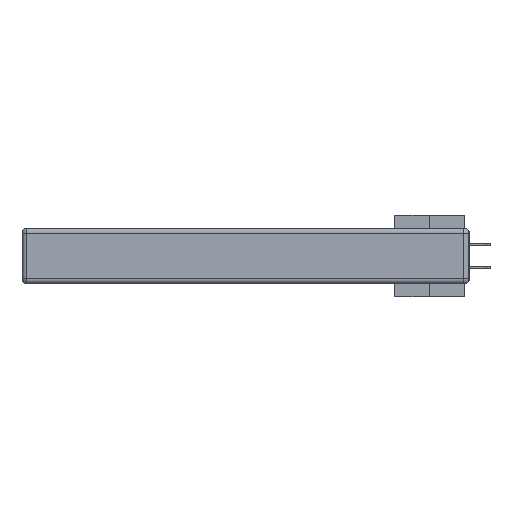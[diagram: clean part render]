
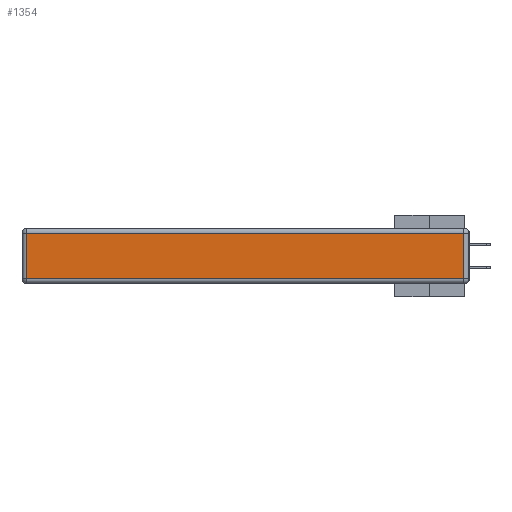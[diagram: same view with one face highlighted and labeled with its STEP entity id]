
A CAD part, left-side view. The second image highlights one B-rep face of the part: STEP entity #1354.
In plain terms, the highlighted planar face has unit normal (-1, 0, 0).
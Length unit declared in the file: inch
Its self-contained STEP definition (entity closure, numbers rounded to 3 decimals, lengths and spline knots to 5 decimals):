
#1354 = ADVANCED_FACE ( 'NONE', ( #19549 ), #22394, .T. ) ;
#1732 = EDGE_CURVE ( 'NONE', #22104, #39568, #37034, .T. ) ;
#2135 = VECTOR ( 'NONE', #3026, 39.37008 ) ;
#3026 = DIRECTION ( 'NONE',  ( 0., 1., 0. ) ) ;
#4450 = CARTESIAN_POINT ( 'NONE',  ( 0., 0.03, -0.313 ) ) ;
#4521 = CARTESIAN_POINT ( 'NONE',  ( 0., 2.72, -0.343 ) ) ;
#7604 = VERTEX_POINT ( 'NONE', #21074 ) ;
#8229 = AXIS2_PLACEMENT_3D ( 'NONE', #32051, #25881, #12905 ) ;
#12905 = DIRECTION ( 'NONE',  ( 0., 0., 1. ) ) ;
#13509 = VECTOR ( 'NONE', #14824, 39.37008 ) ;
#14205 = EDGE_CURVE ( 'NONE', #39568, #21050, #15308, .T. ) ;
#14693 = ORIENTED_EDGE ( 'NONE', *, *, #22444, .T. ) ;
#14824 = DIRECTION ( 'NONE',  ( 0., -1., 0. ) ) ;
#15308 = LINE ( 'NONE', #20934, #35846 ) ;
#17295 = DIRECTION ( 'NONE',  ( 0., 0., 1. ) ) ;
#17671 = CARTESIAN_POINT ( 'NONE',  ( 0., 0., -0.313 ) ) ;
#19263 = CARTESIAN_POINT ( 'NONE',  ( 0., 0.03, -0.03 ) ) ;
#19549 = FACE_OUTER_BOUND ( 'NONE', #19944, .T. ) ;
#19944 = EDGE_LOOP ( 'NONE', ( #39449, #34553, #14693, #27060 ) ) ;
#20934 = CARTESIAN_POINT ( 'NONE',  ( 0., 0.03, -0.343 ) ) ;
#21050 = VERTEX_POINT ( 'NONE', #19263 ) ;
#21074 = CARTESIAN_POINT ( 'NONE',  ( 0., 2.72, -0.03 ) ) ;
#22104 = VERTEX_POINT ( 'NONE', #36295 ) ;
#22394 = PLANE ( 'NONE',  #8229 ) ;
#22444 = EDGE_CURVE ( 'NONE', #21050, #7604, #39155, .T. ) ;
#23056 = VECTOR ( 'NONE', #29343, 39.37008 ) ;
#24532 = LINE ( 'NONE', #4521, #23056 ) ;
#25881 = DIRECTION ( 'NONE',  ( -1., 0., 0. ) ) ;
#27060 = ORIENTED_EDGE ( 'NONE', *, *, #31257, .T. ) ;
#28526 = CARTESIAN_POINT ( 'NONE',  ( 0., 2.75, -0.03 ) ) ;
#29343 = DIRECTION ( 'NONE',  ( 0., 0., -1. ) ) ;
#31257 = EDGE_CURVE ( 'NONE', #7604, #22104, #24532, .T. ) ;
#32051 = CARTESIAN_POINT ( 'NONE',  ( 0., 0., -0.343 ) ) ;
#34553 = ORIENTED_EDGE ( 'NONE', *, *, #14205, .T. ) ;
#35846 = VECTOR ( 'NONE', #17295, 39.37008 ) ;
#36295 = CARTESIAN_POINT ( 'NONE',  ( 0., 2.72, -0.313 ) ) ;
#37034 = LINE ( 'NONE', #17671, #13509 ) ;
#39155 = LINE ( 'NONE', #28526, #2135 ) ;
#39449 = ORIENTED_EDGE ( 'NONE', *, *, #1732, .T. ) ;
#39568 = VERTEX_POINT ( 'NONE', #4450 ) ;
